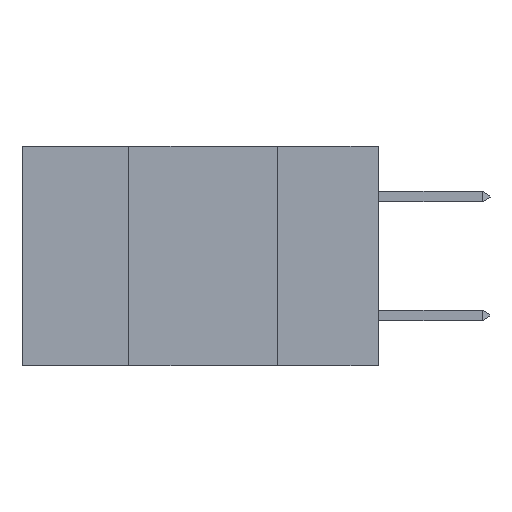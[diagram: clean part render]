
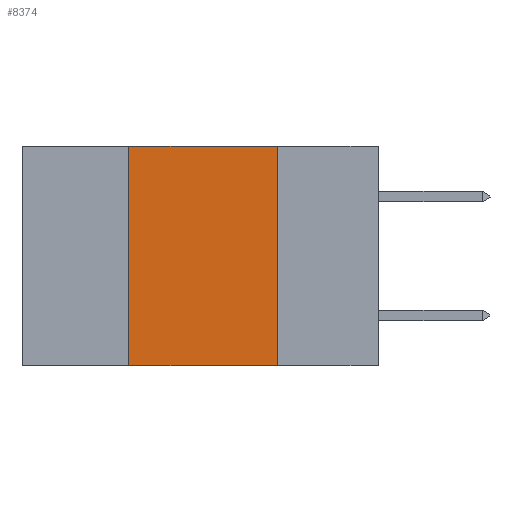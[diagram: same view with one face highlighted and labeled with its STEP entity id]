
A CAD part, left-side view. The second image highlights one B-rep face of the part: STEP entity #8374.
In plain terms, the highlighted planar face has unit normal (-1, 0, 0).
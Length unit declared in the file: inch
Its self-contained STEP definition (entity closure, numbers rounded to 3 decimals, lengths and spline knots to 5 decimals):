
#15 = EDGE_CURVE ( 'NONE', #2773, #15910, #15620, .T. ) ;
#502 = CARTESIAN_POINT ( 'NONE',  ( 0., 0.17, -0.37 ) ) ;
#1964 = CARTESIAN_POINT ( 'NONE',  ( 0., 0.42, 0. ) ) ;
#2207 = CARTESIAN_POINT ( 'NONE',  ( 0., 0.6, -0.37 ) ) ;
#2294 = CARTESIAN_POINT ( 'NONE',  ( 0., 0.42, 0. ) ) ;
#2773 = VERTEX_POINT ( 'NONE', #21869 ) ;
#3621 = PLANE ( 'NONE',  #7976 ) ;
#4123 = ORIENTED_EDGE ( 'NONE', *, *, #18096, .F. ) ;
#4494 = VECTOR ( 'NONE', #15358, 39.37008 ) ;
#5281 = CARTESIAN_POINT ( 'NONE',  ( 0., 0.17, 0. ) ) ;
#6270 = LINE ( 'NONE', #21701, #15011 ) ;
#7711 = VERTEX_POINT ( 'NONE', #502 ) ;
#7976 = AXIS2_PLACEMENT_3D ( 'NONE', #17287, #8622, #11495 ) ;
#8374 = ADVANCED_FACE ( 'NONE', ( #17137 ), #3621, .F. ) ;
#8622 = DIRECTION ( 'NONE',  ( 1., 0., 0. ) ) ;
#11057 = VECTOR ( 'NONE', #14054, 39.37008 ) ;
#11495 = DIRECTION ( 'NONE',  ( 0., 0., -1. ) ) ;
#12453 = LINE ( 'NONE', #2207, #21440 ) ;
#13659 = CARTESIAN_POINT ( 'NONE',  ( 0., 0.6, 0. ) ) ;
#13832 = LINE ( 'NONE', #13659, #4494 ) ;
#14054 = DIRECTION ( 'NONE',  ( 0., 0., 1. ) ) ;
#14279 = ORIENTED_EDGE ( 'NONE', *, *, #20796, .F. ) ;
#14554 = DIRECTION ( 'NONE',  ( 0., -1., 0. ) ) ;
#15011 = VECTOR ( 'NONE', #20029, 39.37008 ) ;
#15358 = DIRECTION ( 'NONE',  ( 0., -1., 0. ) ) ;
#15620 = LINE ( 'NONE', #2294, #11057 ) ;
#15910 = VERTEX_POINT ( 'NONE', #1964 ) ;
#15988 = ORIENTED_EDGE ( 'NONE', *, *, #15, .F. ) ;
#17137 = FACE_OUTER_BOUND ( 'NONE', #19491, .T. ) ;
#17287 = CARTESIAN_POINT ( 'NONE',  ( 0., 0.6, 0. ) ) ;
#18096 = EDGE_CURVE ( 'NONE', #19030, #7711, #6270, .T. ) ;
#19030 = VERTEX_POINT ( 'NONE', #5281 ) ;
#19403 = ORIENTED_EDGE ( 'NONE', *, *, #21481, .T. ) ;
#19491 = EDGE_LOOP ( 'NONE', ( #4123, #14279, #15988, #19403 ) ) ;
#20029 = DIRECTION ( 'NONE',  ( 0., 0., -1. ) ) ;
#20796 = EDGE_CURVE ( 'NONE', #15910, #19030, #13832, .T. ) ;
#21440 = VECTOR ( 'NONE', #14554, 39.37008 ) ;
#21481 = EDGE_CURVE ( 'NONE', #2773, #7711, #12453, .T. ) ;
#21701 = CARTESIAN_POINT ( 'NONE',  ( 0., 0.17, 0. ) ) ;
#21869 = CARTESIAN_POINT ( 'NONE',  ( 0., 0.42, -0.37 ) ) ;
